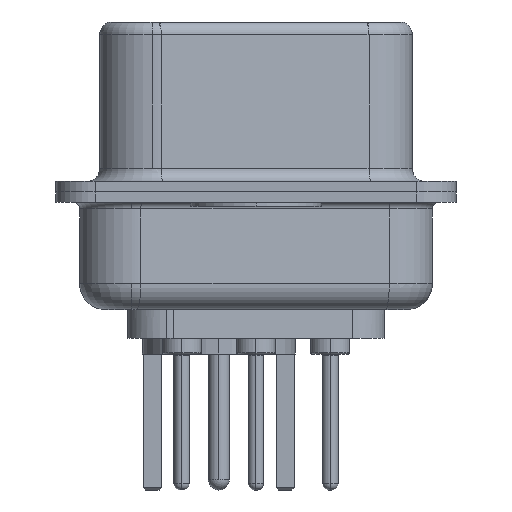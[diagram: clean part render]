
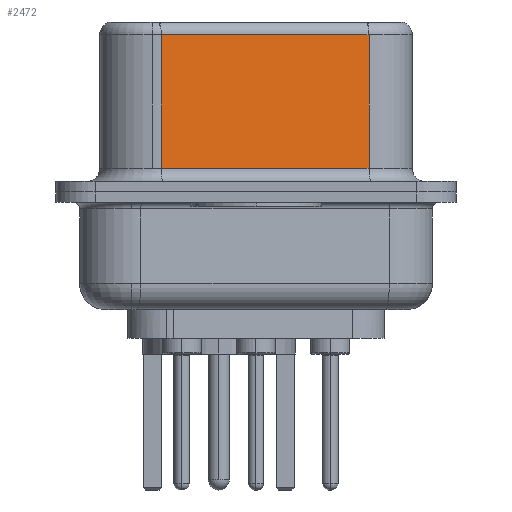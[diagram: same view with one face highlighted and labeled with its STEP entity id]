
A CAD part, left-side view. The second image highlights one B-rep face of the part: STEP entity #2472.
In plain terms, the highlighted planar face has unit normal (-0.985, -0.174, 0).
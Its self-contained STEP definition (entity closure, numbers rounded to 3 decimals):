
#25 = AXIS2_PLACEMENT_3D ( 'NONE', #27260, #10472, #21142 ) ;
#1144 = VECTOR ( 'NONE', #3126, 1000. ) ;
#2351 = DIRECTION ( 'NONE',  ( -0.174, 0.985, 0. ) ) ;
#2472 = ADVANCED_FACE ( 'NONE', ( #8909 ), #9978, .F. ) ;
#3062 = VECTOR ( 'NONE', #2351, 1000. ) ;
#3126 = DIRECTION ( 'NONE',  ( 0., 0., -1. ) ) ;
#3517 = ORIENTED_EDGE ( 'NONE', *, *, #20880, .T. ) ;
#5171 = CARTESIAN_POINT ( 'NONE',  ( 5.132, -4.322, 6.02 ) ) ;
#6579 = VERTEX_POINT ( 'NONE', #14394 ) ;
#8909 = FACE_OUTER_BOUND ( 'NONE', #11982, .T. ) ;
#9101 = CARTESIAN_POINT ( 'NONE',  ( 5.132, -4.322, 6.52 ) ) ;
#9491 = LINE ( 'NONE', #10450, #26591 ) ;
#9978 = PLANE ( 'NONE',  #25 ) ;
#10299 = ORIENTED_EDGE ( 'NONE', *, *, #14932, .F. ) ;
#10450 = CARTESIAN_POINT ( 'NONE',  ( 5.132, -4.322, 0.9 ) ) ;
#10472 = DIRECTION ( 'NONE',  ( 0.985, 0.174, 0. ) ) ;
#10671 = CARTESIAN_POINT ( 'NONE',  ( 5.132, -4.322, 0.9 ) ) ;
#11319 = VERTEX_POINT ( 'NONE', #5171 ) ;
#11894 = VECTOR ( 'NONE', #25331, 1000. ) ;
#11982 = EDGE_LOOP ( 'NONE', ( #10299, #3517, #19533, #12456 ) ) ;
#12456 = ORIENTED_EDGE ( 'NONE', *, *, #13374, .T. ) ;
#12765 = DIRECTION ( 'NONE',  ( 0.174, -0.985, 0. ) ) ;
#13374 = EDGE_CURVE ( 'NONE', #19510, #20617, #9491, .T. ) ;
#14394 = CARTESIAN_POINT ( 'NONE',  ( 3.73, 3.628, 6.02 ) ) ;
#14932 = EDGE_CURVE ( 'NONE', #11319, #20617, #19582, .T. ) ;
#18936 = LINE ( 'NONE', #26371, #1144 ) ;
#19510 = VERTEX_POINT ( 'NONE', #24422 ) ;
#19533 = ORIENTED_EDGE ( 'NONE', *, *, #23067, .T. ) ;
#19582 = LINE ( 'NONE', #9101, #11894 ) ;
#20617 = VERTEX_POINT ( 'NONE', #10671 ) ;
#20880 = EDGE_CURVE ( 'NONE', #11319, #6579, #22246, .T. ) ;
#21142 = DIRECTION ( 'NONE',  ( -0.174, 0.985, 0. ) ) ;
#22246 = LINE ( 'NONE', #23141, #3062 ) ;
#23067 = EDGE_CURVE ( 'NONE', #6579, #19510, #18936, .T. ) ;
#23141 = CARTESIAN_POINT ( 'NONE',  ( 5.132, -4.322, 6.02 ) ) ;
#24422 = CARTESIAN_POINT ( 'NONE',  ( 3.73, 3.628, 0.9 ) ) ;
#25331 = DIRECTION ( 'NONE',  ( 0., 0., -1. ) ) ;
#26371 = CARTESIAN_POINT ( 'NONE',  ( 3.73, 3.628, 6.52 ) ) ;
#26591 = VECTOR ( 'NONE', #12765, 1000. ) ;
#27260 = CARTESIAN_POINT ( 'NONE',  ( 5.132, -4.322, 6.52 ) ) ;
